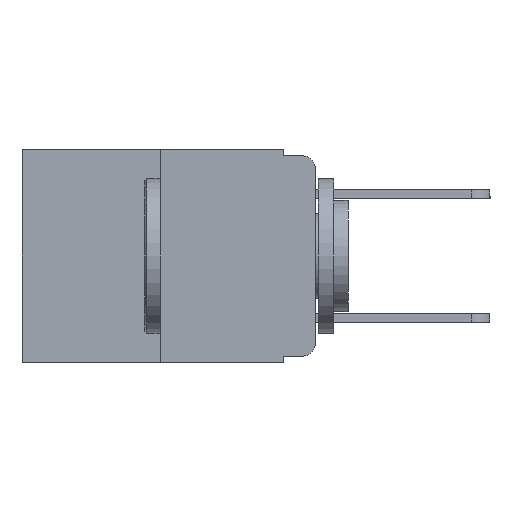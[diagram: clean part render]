
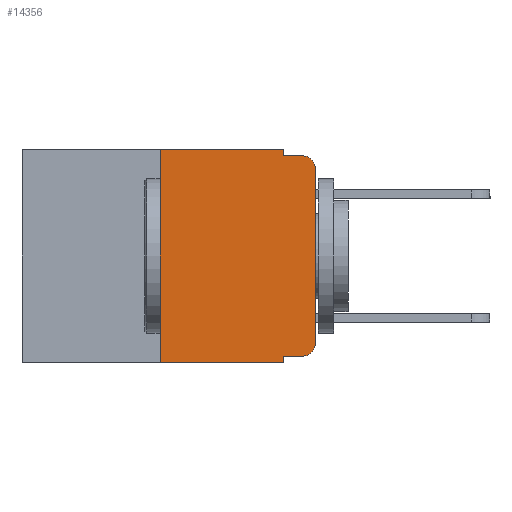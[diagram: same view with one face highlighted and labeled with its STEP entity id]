
A CAD part, left-side view. The second image highlights one B-rep face of the part: STEP entity #14356.
In plain terms, the highlighted planar face has unit normal (-1, 0, 0).
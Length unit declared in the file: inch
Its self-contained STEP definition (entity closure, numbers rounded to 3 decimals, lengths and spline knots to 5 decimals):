
#183 = VERTEX_POINT ( 'NONE', #26370 ) ;
#305 = CARTESIAN_POINT ( 'NONE',  ( 0., 0.051, 0. ) ) ;
#493 = VERTEX_POINT ( 'NONE', #23827 ) ;
#583 = CARTESIAN_POINT ( 'NONE',  ( 0., 0., -0.03 ) ) ;
#642 = CARTESIAN_POINT ( 'NONE',  ( 0., 0., 0. ) ) ;
#1162 = ORIENTED_EDGE ( 'NONE', *, *, #11224, .F. ) ;
#1198 = CARTESIAN_POINT ( 'NONE',  ( 0., 0.473, -0.343 ) ) ;
#1240 = EDGE_CURVE ( 'NONE', #11647, #183, #4161, .T. ) ;
#1922 = VERTEX_POINT ( 'NONE', #583 ) ;
#1980 = DIRECTION ( 'NONE',  ( 0., -1., 0. ) ) ;
#2394 = EDGE_CURVE ( 'NONE', #9797, #15241, #16748, .T. ) ;
#2763 = EDGE_CURVE ( 'NONE', #183, #22879, #3437, .T. ) ;
#3437 = LINE ( 'NONE', #7148, #13894 ) ;
#3447 = LINE ( 'NONE', #642, #24498 ) ;
#3480 = VECTOR ( 'NONE', #9668, 39.37008 ) ;
#4161 = LINE ( 'NONE', #12482, #3480 ) ;
#4162 = ORIENTED_EDGE ( 'NONE', *, *, #1240, .F. ) ;
#4238 = PLANE ( 'NONE',  #20186 ) ;
#4321 = LINE ( 'NONE', #12629, #24662 ) ;
#4479 = ORIENTED_EDGE ( 'NONE', *, *, #18037, .F. ) ;
#4519 = EDGE_CURVE ( 'NONE', #1922, #18512, #20404, .T. ) ;
#5367 = VERTEX_POINT ( 'NONE', #26421 ) ;
#5704 = CARTESIAN_POINT ( 'NONE',  ( 0., 0.25, -0.343 ) ) ;
#6301 = CARTESIAN_POINT ( 'NONE',  ( 0., 0.473, 0. ) ) ;
#6397 = DIRECTION ( 'NONE',  ( 1., 0., 0. ) ) ;
#6413 = VERTEX_POINT ( 'NONE', #25869 ) ;
#6923 = CARTESIAN_POINT ( 'NONE',  ( 0., 0.051, -0.01 ) ) ;
#7148 = CARTESIAN_POINT ( 'NONE',  ( 0., 0.051, 0. ) ) ;
#8785 = EDGE_CURVE ( 'NONE', #5367, #1922, #3447, .T. ) ;
#9668 = DIRECTION ( 'NONE',  ( 0., -1., 0. ) ) ;
#9797 = VERTEX_POINT ( 'NONE', #5704 ) ;
#10170 = FACE_OUTER_BOUND ( 'NONE', #14516, .T. ) ;
#11091 = DIRECTION ( 'NONE',  ( 0., -1., 0. ) ) ;
#11224 = EDGE_CURVE ( 'NONE', #9797, #11647, #4321, .T. ) ;
#11353 = VECTOR ( 'NONE', #25196, 39.37008 ) ;
#11417 = ORIENTED_EDGE ( 'NONE', *, *, #22995, .T. ) ;
#11647 = VERTEX_POINT ( 'NONE', #20004 ) ;
#11710 = CARTESIAN_POINT ( 'NONE',  ( 0., 0.051, -0.01 ) ) ;
#12448 = CARTESIAN_POINT ( 'NONE',  ( 0., 0.051, -0.333 ) ) ;
#12482 = CARTESIAN_POINT ( 'NONE',  ( 0., 0.473, 0. ) ) ;
#12518 = DIRECTION ( 'NONE',  ( -1., 0., 0. ) ) ;
#12629 = CARTESIAN_POINT ( 'NONE',  ( 0., 0.25, 0. ) ) ;
#12659 = ORIENTED_EDGE ( 'NONE', *, *, #2763, .F. ) ;
#13238 = DIRECTION ( 'NONE',  ( 0., 0., 1. ) ) ;
#13894 = VECTOR ( 'NONE', #14102, 39.37008 ) ;
#14102 = DIRECTION ( 'NONE',  ( 0., 0., -1. ) ) ;
#14356 = ADVANCED_FACE ( 'NONE', ( #10170 ), #4238, .F. ) ;
#14470 = EDGE_CURVE ( 'NONE', #493, #15241, #19035, .T. ) ;
#14516 = EDGE_LOOP ( 'NONE', ( #18366, #19593, #4479, #12659, #4162, #1162, #23318, #19323, #19939, #11417 ) ) ;
#14664 = DIRECTION ( 'NONE',  ( 0., 0., 1. ) ) ;
#15241 = VERTEX_POINT ( 'NONE', #21904 ) ;
#16748 = LINE ( 'NONE', #1198, #11353 ) ;
#16960 = DIRECTION ( 'NONE',  ( 0., 0., -1. ) ) ;
#17394 = DIRECTION ( 'NONE',  ( 0., 0., -1. ) ) ;
#17545 = DIRECTION ( 'NONE',  ( -1., 0., 0. ) ) ;
#18037 = EDGE_CURVE ( 'NONE', #22879, #18512, #22148, .T. ) ;
#18335 = CARTESIAN_POINT ( 'NONE',  ( 0., 0.02, -0.03 ) ) ;
#18366 = ORIENTED_EDGE ( 'NONE', *, *, #8785, .T. ) ;
#18512 = VERTEX_POINT ( 'NONE', #26432 ) ;
#19035 = LINE ( 'NONE', #305, #23653 ) ;
#19323 = ORIENTED_EDGE ( 'NONE', *, *, #14470, .F. ) ;
#19593 = ORIENTED_EDGE ( 'NONE', *, *, #4519, .T. ) ;
#19939 = ORIENTED_EDGE ( 'NONE', *, *, #22518, .T. ) ;
#20004 = CARTESIAN_POINT ( 'NONE',  ( 0., 0.25, 0. ) ) ;
#20186 = AXIS2_PLACEMENT_3D ( 'NONE', #6301, #6397, #20641 ) ;
#20404 = CIRCLE ( 'NONE', #24945, 0.02 ) ;
#20641 = DIRECTION ( 'NONE',  ( 0., 0., -1. ) ) ;
#21544 = VECTOR ( 'NONE', #11091, 39.37008 ) ;
#21812 = AXIS2_PLACEMENT_3D ( 'NONE', #24470, #12518, #26442 ) ;
#21904 = CARTESIAN_POINT ( 'NONE',  ( 0., 0.051, -0.343 ) ) ;
#22148 = LINE ( 'NONE', #6923, #21544 ) ;
#22278 = LINE ( 'NONE', #12448, #25637 ) ;
#22518 = EDGE_CURVE ( 'NONE', #493, #6413, #22278, .T. ) ;
#22879 = VERTEX_POINT ( 'NONE', #11710 ) ;
#22995 = EDGE_CURVE ( 'NONE', #6413, #5367, #24382, .T. ) ;
#23318 = ORIENTED_EDGE ( 'NONE', *, *, #2394, .T. ) ;
#23653 = VECTOR ( 'NONE', #16960, 39.37008 ) ;
#23827 = CARTESIAN_POINT ( 'NONE',  ( 0., 0.051, -0.333 ) ) ;
#24382 = CIRCLE ( 'NONE', #21812, 0.02 ) ;
#24470 = CARTESIAN_POINT ( 'NONE',  ( 0., 0.02, -0.313 ) ) ;
#24498 = VECTOR ( 'NONE', #13238, 39.37008 ) ;
#24662 = VECTOR ( 'NONE', #14664, 39.37008 ) ;
#24945 = AXIS2_PLACEMENT_3D ( 'NONE', #18335, #17545, #17394 ) ;
#25196 = DIRECTION ( 'NONE',  ( 0., -1., 0. ) ) ;
#25637 = VECTOR ( 'NONE', #1980, 39.37008 ) ;
#25869 = CARTESIAN_POINT ( 'NONE',  ( 0., 0.02, -0.333 ) ) ;
#26370 = CARTESIAN_POINT ( 'NONE',  ( 0., 0.051, 0. ) ) ;
#26421 = CARTESIAN_POINT ( 'NONE',  ( 0., 0., -0.313 ) ) ;
#26432 = CARTESIAN_POINT ( 'NONE',  ( 0., 0.02, -0.01 ) ) ;
#26442 = DIRECTION ( 'NONE',  ( 0., 0., -1. ) ) ;
